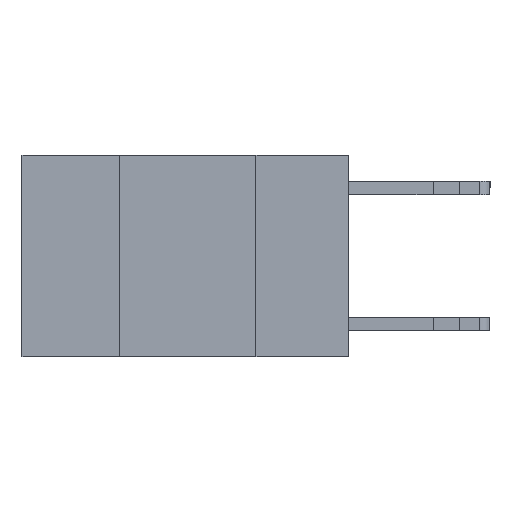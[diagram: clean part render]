
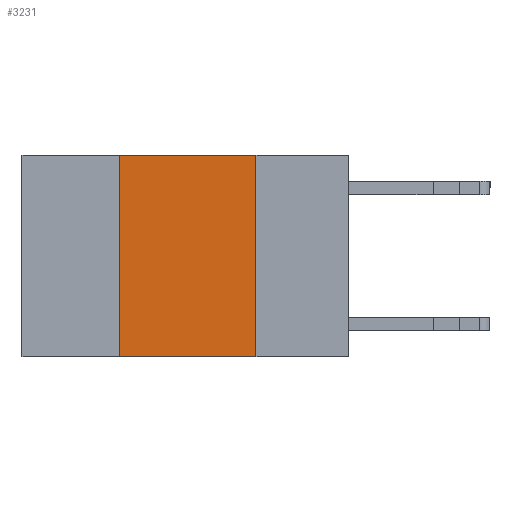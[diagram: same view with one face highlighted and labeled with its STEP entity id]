
A CAD part, left-side view. The second image highlights one B-rep face of the part: STEP entity #3231.
In plain terms, the highlighted planar face has unit normal (-1, 0, 0).
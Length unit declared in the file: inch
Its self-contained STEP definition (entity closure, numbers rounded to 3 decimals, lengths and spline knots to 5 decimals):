
#116 = CARTESIAN_POINT ( 'NONE',  ( 0., 0.6, 0. ) ) ;
#297 = LINE ( 'NONE', #116, #8448 ) ;
#647 = CARTESIAN_POINT ( 'NONE',  ( 0., 0.42, -0.37 ) ) ;
#1976 = CARTESIAN_POINT ( 'NONE',  ( 0., 0.17, 0. ) ) ;
#2689 = VERTEX_POINT ( 'NONE', #1976 ) ;
#3069 = EDGE_CURVE ( 'NONE', #7671, #16071, #3748, .T. ) ;
#3106 = VERTEX_POINT ( 'NONE', #7106 ) ;
#3231 = ADVANCED_FACE ( 'NONE', ( #13633 ), #5033, .F. ) ;
#3597 = CARTESIAN_POINT ( 'NONE',  ( 0., 0.6, 0. ) ) ;
#3748 = LINE ( 'NONE', #10774, #18319 ) ;
#4363 = CARTESIAN_POINT ( 'NONE',  ( 0., 0.17, 0. ) ) ;
#4940 = DIRECTION ( 'NONE',  ( 1., 0., 0. ) ) ;
#5033 = PLANE ( 'NONE',  #11392 ) ;
#5137 = DIRECTION ( 'NONE',  ( 0., 0., -1. ) ) ;
#5696 = EDGE_CURVE ( 'NONE', #2689, #16071, #5836, .T. ) ;
#5836 = LINE ( 'NONE', #4363, #6528 ) ;
#5980 = CARTESIAN_POINT ( 'NONE',  ( 0., 0.17, -0.37 ) ) ;
#6528 = VECTOR ( 'NONE', #11571, 39.37008 ) ;
#6970 = EDGE_CURVE ( 'NONE', #3106, #2689, #297, .T. ) ;
#7106 = CARTESIAN_POINT ( 'NONE',  ( 0., 0.42, 0. ) ) ;
#7671 = VERTEX_POINT ( 'NONE', #647 ) ;
#7752 = EDGE_LOOP ( 'NONE', ( #12731, #14130, #16179, #11127 ) ) ;
#8448 = VECTOR ( 'NONE', #11846, 39.37008 ) ;
#10509 = CARTESIAN_POINT ( 'NONE',  ( 0., 0.42, 0. ) ) ;
#10774 = CARTESIAN_POINT ( 'NONE',  ( 0., 0.6, -0.37 ) ) ;
#11019 = VECTOR ( 'NONE', #12017, 39.37008 ) ;
#11127 = ORIENTED_EDGE ( 'NONE', *, *, #3069, .T. ) ;
#11392 = AXIS2_PLACEMENT_3D ( 'NONE', #3597, #4940, #5137 ) ;
#11571 = DIRECTION ( 'NONE',  ( 0., 0., -1. ) ) ;
#11846 = DIRECTION ( 'NONE',  ( 0., -1., 0. ) ) ;
#12017 = DIRECTION ( 'NONE',  ( 0., 0., 1. ) ) ;
#12731 = ORIENTED_EDGE ( 'NONE', *, *, #5696, .F. ) ;
#13224 = EDGE_CURVE ( 'NONE', #7671, #3106, #14912, .T. ) ;
#13633 = FACE_OUTER_BOUND ( 'NONE', #7752, .T. ) ;
#14130 = ORIENTED_EDGE ( 'NONE', *, *, #6970, .F. ) ;
#14912 = LINE ( 'NONE', #10509, #11019 ) ;
#16071 = VERTEX_POINT ( 'NONE', #5980 ) ;
#16179 = ORIENTED_EDGE ( 'NONE', *, *, #13224, .F. ) ;
#16497 = DIRECTION ( 'NONE',  ( 0., -1., 0. ) ) ;
#18319 = VECTOR ( 'NONE', #16497, 39.37008 ) ;
